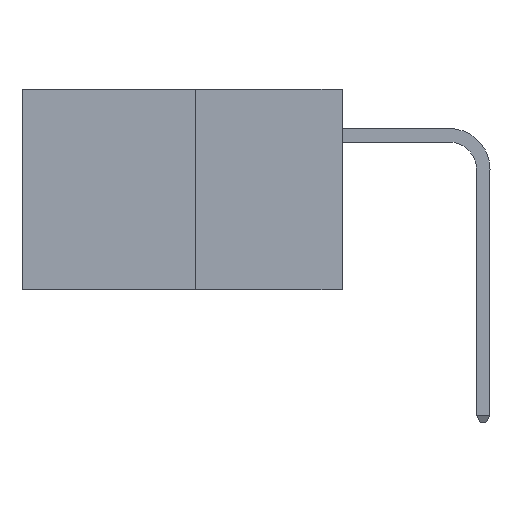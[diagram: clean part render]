
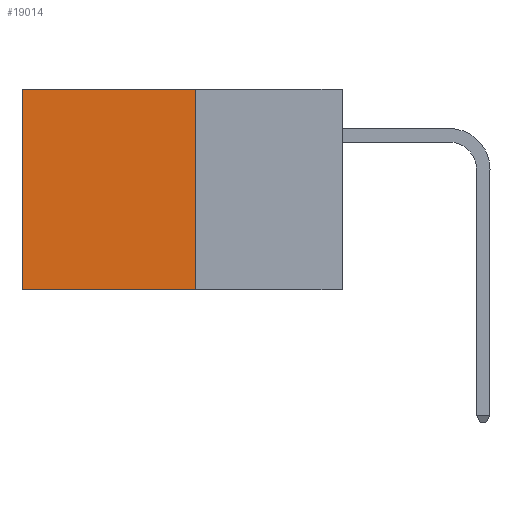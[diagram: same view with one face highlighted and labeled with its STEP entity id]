
A CAD part, left-side view. The second image highlights one B-rep face of the part: STEP entity #19014.
In plain terms, the highlighted planar face has unit normal (-1, 0, 0).
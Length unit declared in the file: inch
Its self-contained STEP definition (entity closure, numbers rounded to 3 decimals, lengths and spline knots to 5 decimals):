
#320 = VERTEX_POINT ( 'NONE', #25157 ) ;
#804 = ORIENTED_EDGE ( 'NONE', *, *, #17639, .F. ) ;
#1417 = VECTOR ( 'NONE', #32248, 39.37008 ) ;
#3509 = LINE ( 'NONE', #24018, #30234 ) ;
#4426 = PLANE ( 'NONE',  #19320 ) ;
#6225 = LINE ( 'NONE', #22011, #26053 ) ;
#6469 = VERTEX_POINT ( 'NONE', #10683 ) ;
#6493 = DIRECTION ( 'NONE',  ( 0., 1., 0. ) ) ;
#6666 = EDGE_CURVE ( 'NONE', #6469, #30267, #24831, .T. ) ;
#7580 = ORIENTED_EDGE ( 'NONE', *, *, #6666, .F. ) ;
#8288 = DIRECTION ( 'NONE',  ( 0., 0., -1. ) ) ;
#8527 = CARTESIAN_POINT ( 'NONE',  ( 0.277, 0.27, -0.37 ) ) ;
#9696 = EDGE_CURVE ( 'NONE', #320, #26292, #28127, .T. ) ;
#9773 = CARTESIAN_POINT ( 'NONE',  ( 0.277, 0.27, -0.37 ) ) ;
#10330 = ORIENTED_EDGE ( 'NONE', *, *, #20727, .T. ) ;
#10683 = CARTESIAN_POINT ( 'NONE',  ( 0.277, 0.27, 0. ) ) ;
#11371 = DIRECTION ( 'NONE',  ( 0., 1., 0. ) ) ;
#12107 = CARTESIAN_POINT ( 'NONE',  ( 0.277, 0.59, -0.37 ) ) ;
#12393 = DIRECTION ( 'NONE',  ( 0., 0., -1. ) ) ;
#13928 = FACE_OUTER_BOUND ( 'NONE', #18592, .T. ) ;
#17639 = EDGE_CURVE ( 'NONE', #30267, #26292, #6225, .T. ) ;
#18067 = VECTOR ( 'NONE', #8288, 39.37008 ) ;
#18592 = EDGE_LOOP ( 'NONE', ( #18631, #804, #7580, #10330 ) ) ;
#18631 = ORIENTED_EDGE ( 'NONE', *, *, #9696, .T. ) ;
#19014 = ADVANCED_FACE ( 'NONE', ( #13928 ), #4426, .F. ) ;
#19320 = AXIS2_PLACEMENT_3D ( 'NONE', #9773, #27758, #12393 ) ;
#20727 = EDGE_CURVE ( 'NONE', #6469, #320, #3509, .T. ) ;
#22011 = CARTESIAN_POINT ( 'NONE',  ( 0.277, 0.27, -0.37 ) ) ;
#22872 = CARTESIAN_POINT ( 'NONE',  ( 0.277, 0.59, -0.37 ) ) ;
#24018 = CARTESIAN_POINT ( 'NONE',  ( 0.277, 0.27, 0. ) ) ;
#24831 = LINE ( 'NONE', #8527, #18067 ) ;
#25157 = CARTESIAN_POINT ( 'NONE',  ( 0.277, 0.59, 0. ) ) ;
#26053 = VECTOR ( 'NONE', #6493, 39.37008 ) ;
#26292 = VERTEX_POINT ( 'NONE', #12107 ) ;
#27758 = DIRECTION ( 'NONE',  ( 1., 0., 0. ) ) ;
#28127 = LINE ( 'NONE', #22872, #1417 ) ;
#30234 = VECTOR ( 'NONE', #11371, 39.37008 ) ;
#30267 = VERTEX_POINT ( 'NONE', #32832 ) ;
#32248 = DIRECTION ( 'NONE',  ( 0., 0., -1. ) ) ;
#32832 = CARTESIAN_POINT ( 'NONE',  ( 0.277, 0.27, -0.37 ) ) ;
